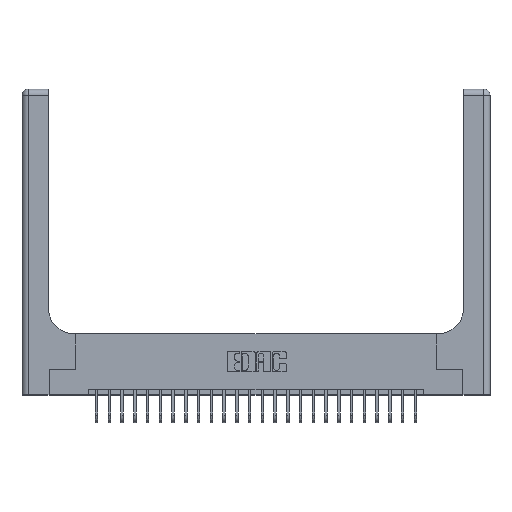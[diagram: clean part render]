
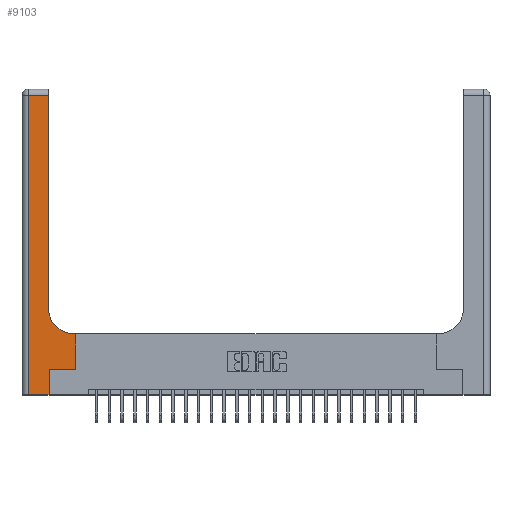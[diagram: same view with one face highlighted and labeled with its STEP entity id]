
A CAD part, top view. The second image highlights one B-rep face of the part: STEP entity #9103.
In plain terms, the highlighted planar face has unit normal (0, 0, 1).
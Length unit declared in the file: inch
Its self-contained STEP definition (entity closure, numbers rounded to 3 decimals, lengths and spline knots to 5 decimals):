
#237 = ORIENTED_EDGE ( 'NONE', *, *, #5683, .T. ) ;
#756 = EDGE_CURVE ( 'NONE', #23341, #9538, #3688, .T. ) ;
#858 = EDGE_CURVE ( 'NONE', #9538, #14561, #11828, .T. ) ;
#945 = ORIENTED_EDGE ( 'NONE', *, *, #6393, .T. ) ;
#970 = AXIS2_PLACEMENT_3D ( 'NONE', #2615, #7840, #21195 ) ;
#1324 = VERTEX_POINT ( 'NONE', #9593 ) ;
#1340 = DIRECTION ( 'NONE',  ( 1., 0., 0. ) ) ;
#1414 = AXIS2_PLACEMENT_3D ( 'NONE', #3449, #1647, #18625 ) ;
#1647 = DIRECTION ( 'NONE',  ( 0., 0., -1. ) ) ;
#1702 = CARTESIAN_POINT ( 'NONE',  ( 0.26, 3., 0.37 ) ) ;
#1723 = CARTESIAN_POINT ( 'NONE',  ( 0.06, 0., 0.37 ) ) ;
#1815 = EDGE_LOOP ( 'NONE', ( #945, #23587, #3291, #237, #14805, #18290, #6821, #17941, #16047 ) ) ;
#1978 = LINE ( 'NONE', #20550, #3585 ) ;
#2385 = PLANE ( 'NONE',  #970 ) ;
#2456 = VECTOR ( 'NONE', #3268, 39.37008 ) ;
#2615 = CARTESIAN_POINT ( 'NONE',  ( 0., 3., 0.37 ) ) ;
#2645 = CARTESIAN_POINT ( 'NONE',  ( 0.265, 0., 0.37 ) ) ;
#2915 = LINE ( 'NONE', #6440, #10503 ) ;
#3268 = DIRECTION ( 'NONE',  ( 0., 1., 0. ) ) ;
#3291 = ORIENTED_EDGE ( 'NONE', *, *, #19387, .T. ) ;
#3449 = CARTESIAN_POINT ( 'NONE',  ( 0.51, 0.85, 0.37 ) ) ;
#3585 = VECTOR ( 'NONE', #3911, 39.37008 ) ;
#3681 = VECTOR ( 'NONE', #16560, 39.37008 ) ;
#3688 = LINE ( 'NONE', #7327, #19222 ) ;
#3911 = DIRECTION ( 'NONE',  ( 0., 1., 0. ) ) ;
#4821 = CARTESIAN_POINT ( 'NONE',  ( 0.528, 0.25, 0.37 ) ) ;
#5683 = EDGE_CURVE ( 'NONE', #20773, #20900, #9165, .T. ) ;
#5711 = CARTESIAN_POINT ( 'NONE',  ( 0.26, 2.94, 0.37 ) ) ;
#6306 = EDGE_CURVE ( 'NONE', #20835, #21734, #9089, .T. ) ;
#6393 = EDGE_CURVE ( 'NONE', #14561, #8558, #16593, .T. ) ;
#6440 = CARTESIAN_POINT ( 'NONE',  ( 0.06, 3., 0.37 ) ) ;
#6506 = VECTOR ( 'NONE', #19499, 39.37008 ) ;
#6821 = ORIENTED_EDGE ( 'NONE', *, *, #9258, .T. ) ;
#7327 = CARTESIAN_POINT ( 'NONE',  ( 0.26, 0.6, 0.37 ) ) ;
#7840 = DIRECTION ( 'NONE',  ( 0., 0., -1. ) ) ;
#8558 = VERTEX_POINT ( 'NONE', #5711 ) ;
#8813 = LINE ( 'NONE', #4821, #6506 ) ;
#9089 = LINE ( 'NONE', #16125, #19906 ) ;
#9103 = ADVANCED_FACE ( 'NONE', ( #23023 ), #2385, .F. ) ;
#9165 = LINE ( 'NONE', #13149, #3681 ) ;
#9258 = EDGE_CURVE ( 'NONE', #21734, #23341, #8813, .T. ) ;
#9538 = VERTEX_POINT ( 'NONE', #13620 ) ;
#9593 = CARTESIAN_POINT ( 'NONE',  ( 0.06, 2.94, 0.37 ) ) ;
#10503 = VECTOR ( 'NONE', #23452, 39.37008 ) ;
#11075 = CARTESIAN_POINT ( 'NONE',  ( 0., 2.94, 0.37 ) ) ;
#11828 = CIRCLE ( 'NONE', #1414, 0.25 ) ;
#12789 = EDGE_CURVE ( 'NONE', #8558, #1324, #22509, .T. ) ;
#12908 = DIRECTION ( 'NONE',  ( -1., 0., 0. ) ) ;
#13149 = CARTESIAN_POINT ( 'NONE',  ( 0., 0., 0.37 ) ) ;
#13620 = CARTESIAN_POINT ( 'NONE',  ( 0.51, 0.6, 0.37 ) ) ;
#14169 = CARTESIAN_POINT ( 'NONE',  ( 0.528, 0.6, 0.37 ) ) ;
#14214 = VECTOR ( 'NONE', #12908, 39.37008 ) ;
#14561 = VERTEX_POINT ( 'NONE', #18957 ) ;
#14805 = ORIENTED_EDGE ( 'NONE', *, *, #20483, .T. ) ;
#16047 = ORIENTED_EDGE ( 'NONE', *, *, #858, .T. ) ;
#16125 = CARTESIAN_POINT ( 'NONE',  ( 0.265, 0.25, 0.37 ) ) ;
#16560 = DIRECTION ( 'NONE',  ( 1., 0., 0. ) ) ;
#16593 = LINE ( 'NONE', #1702, #2456 ) ;
#16665 = DIRECTION ( 'NONE',  ( -1., 0., 0. ) ) ;
#17941 = ORIENTED_EDGE ( 'NONE', *, *, #756, .T. ) ;
#18290 = ORIENTED_EDGE ( 'NONE', *, *, #6306, .T. ) ;
#18625 = DIRECTION ( 'NONE',  ( 1., 0., 0. ) ) ;
#18957 = CARTESIAN_POINT ( 'NONE',  ( 0.26, 0.85, 0.37 ) ) ;
#19222 = VECTOR ( 'NONE', #16665, 39.37008 ) ;
#19387 = EDGE_CURVE ( 'NONE', #1324, #20773, #2915, .T. ) ;
#19499 = DIRECTION ( 'NONE',  ( 0., 1., 0. ) ) ;
#19906 = VECTOR ( 'NONE', #1340, 39.37008 ) ;
#20483 = EDGE_CURVE ( 'NONE', #20900, #20835, #1978, .T. ) ;
#20550 = CARTESIAN_POINT ( 'NONE',  ( 0.265, 0., 0.37 ) ) ;
#20773 = VERTEX_POINT ( 'NONE', #1723 ) ;
#20835 = VERTEX_POINT ( 'NONE', #22582 ) ;
#20900 = VERTEX_POINT ( 'NONE', #2645 ) ;
#21195 = DIRECTION ( 'NONE',  ( -1., 0., 0. ) ) ;
#21287 = CARTESIAN_POINT ( 'NONE',  ( 0.528, 0.25, 0.37 ) ) ;
#21734 = VERTEX_POINT ( 'NONE', #21287 ) ;
#22509 = LINE ( 'NONE', #11075, #14214 ) ;
#22582 = CARTESIAN_POINT ( 'NONE',  ( 0.265, 0.25, 0.37 ) ) ;
#23023 = FACE_OUTER_BOUND ( 'NONE', #1815, .T. ) ;
#23341 = VERTEX_POINT ( 'NONE', #14169 ) ;
#23452 = DIRECTION ( 'NONE',  ( 0., -1., 0. ) ) ;
#23587 = ORIENTED_EDGE ( 'NONE', *, *, #12789, .T. ) ;
